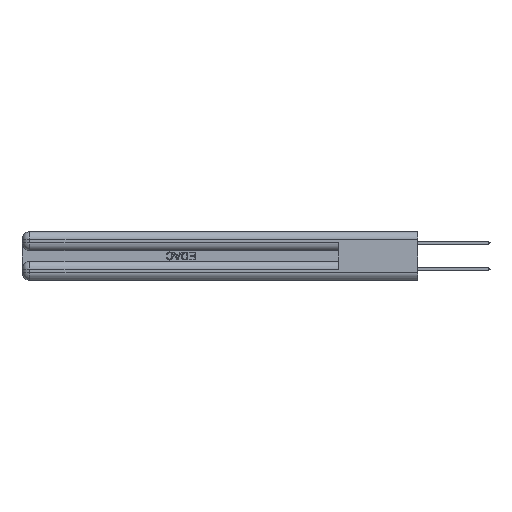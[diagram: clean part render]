
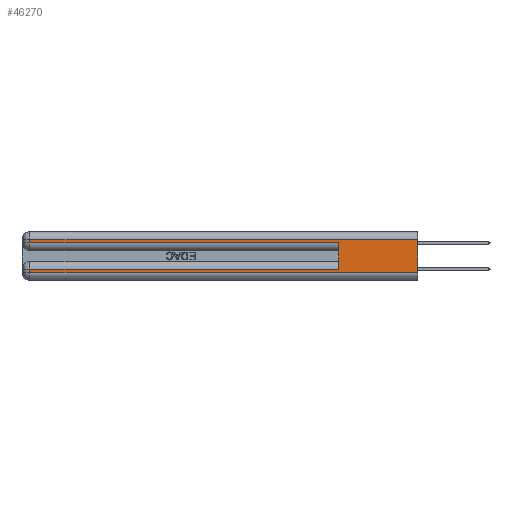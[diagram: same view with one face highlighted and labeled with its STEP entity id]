
A CAD part, left-side view. The second image highlights one B-rep face of the part: STEP entity #46270.
In plain terms, the highlighted planar face has unit normal (-1, 0, 0).
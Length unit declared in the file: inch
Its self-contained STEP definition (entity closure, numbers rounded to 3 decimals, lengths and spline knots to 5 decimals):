
#1334 = CARTESIAN_POINT ( 'NONE',  ( 0., 2.94, 0.085 ) ) ;
#1571 = DIRECTION ( 'NONE',  ( 1., 0., 0. ) ) ;
#2046 = VECTOR ( 'NONE', #31151, 39.37008 ) ;
#2434 = AXIS2_PLACEMENT_3D ( 'NONE', #24019, #1571, #27946 ) ;
#3296 = LINE ( 'NONE', #25047, #31011 ) ;
#3628 = EDGE_LOOP ( 'NONE', ( #4961, #23378, #37711, #9374, #30080, #7433, #8274, #8623 ) ) ;
#3970 = DIRECTION ( 'NONE',  ( 0., 0., -1. ) ) ;
#4219 = EDGE_CURVE ( 'NONE', #15027, #23163, #40047, .T. ) ;
#4768 = CARTESIAN_POINT ( 'NONE',  ( 0., 0., 0.285 ) ) ;
#4961 = ORIENTED_EDGE ( 'NONE', *, *, #28759, .F. ) ;
#6070 = DIRECTION ( 'NONE',  ( 0., 1., 0. ) ) ;
#7433 = ORIENTED_EDGE ( 'NONE', *, *, #25814, .T. ) ;
#7521 = CARTESIAN_POINT ( 'NONE',  ( 0., 0.6, 0.085 ) ) ;
#8274 = ORIENTED_EDGE ( 'NONE', *, *, #43996, .T. ) ;
#8623 = ORIENTED_EDGE ( 'NONE', *, *, #4219, .T. ) ;
#9374 = ORIENTED_EDGE ( 'NONE', *, *, #42820, .T. ) ;
#12802 = CARTESIAN_POINT ( 'NONE',  ( 0., 0., 0.31 ) ) ;
#14272 = LINE ( 'NONE', #15020, #41834 ) ;
#15020 = CARTESIAN_POINT ( 'NONE',  ( 0., 0., 0.37 ) ) ;
#15027 = VERTEX_POINT ( 'NONE', #15856 ) ;
#15388 = CARTESIAN_POINT ( 'NONE',  ( 0., 0., 0.06 ) ) ;
#15402 = DIRECTION ( 'NONE',  ( 0., 0., -1. ) ) ;
#15676 = LINE ( 'NONE', #45189, #44361 ) ;
#15723 = LINE ( 'NONE', #34809, #43228 ) ;
#15856 = CARTESIAN_POINT ( 'NONE',  ( 0., 2.94, 0.06 ) ) ;
#16581 = VERTEX_POINT ( 'NONE', #17724 ) ;
#16589 = DIRECTION ( 'NONE',  ( 0., 1., 0. ) ) ;
#17169 = VECTOR ( 'NONE', #43447, 39.37008 ) ;
#17310 = CARTESIAN_POINT ( 'NONE',  ( 0., 2.94, 0.37 ) ) ;
#17724 = CARTESIAN_POINT ( 'NONE',  ( 0., 0., 0.31 ) ) ;
#20739 = EDGE_CURVE ( 'NONE', #16581, #26210, #39773, .T. ) ;
#21359 = VERTEX_POINT ( 'NONE', #27719 ) ;
#23163 = VERTEX_POINT ( 'NONE', #15388 ) ;
#23378 = ORIENTED_EDGE ( 'NONE', *, *, #20739, .T. ) ;
#23941 = EDGE_CURVE ( 'NONE', #26210, #21359, #26007, .T. ) ;
#24019 = CARTESIAN_POINT ( 'NONE',  ( 0., 0., 0.37 ) ) ;
#24650 = CARTESIAN_POINT ( 'NONE',  ( 0., 0., 0.06 ) ) ;
#25047 = CARTESIAN_POINT ( 'NONE',  ( 0., 0., 0.085 ) ) ;
#25814 = EDGE_CURVE ( 'NONE', #48408, #33801, #3296, .T. ) ;
#26007 = LINE ( 'NONE', #17310, #17169 ) ;
#26210 = VERTEX_POINT ( 'NONE', #27298 ) ;
#27298 = CARTESIAN_POINT ( 'NONE',  ( 0., 2.94, 0.31 ) ) ;
#27719 = CARTESIAN_POINT ( 'NONE',  ( 0., 2.94, 0.285 ) ) ;
#27946 = DIRECTION ( 'NONE',  ( 0., 0., -1. ) ) ;
#28481 = FACE_OUTER_BOUND ( 'NONE', #3628, .T. ) ;
#28759 = EDGE_CURVE ( 'NONE', #16581, #23163, #14272, .T. ) ;
#29765 = LINE ( 'NONE', #4768, #2046 ) ;
#30080 = ORIENTED_EDGE ( 'NONE', *, *, #43512, .F. ) ;
#30147 = VECTOR ( 'NONE', #43397, 39.37008 ) ;
#31011 = VECTOR ( 'NONE', #6070, 39.37008 ) ;
#31151 = DIRECTION ( 'NONE',  ( 0., -1., 0. ) ) ;
#33801 = VERTEX_POINT ( 'NONE', #1334 ) ;
#34809 = CARTESIAN_POINT ( 'NONE',  ( 0., 0.6, 0.145 ) ) ;
#37660 = CARTESIAN_POINT ( 'NONE',  ( 0., 0.6, 0.285 ) ) ;
#37711 = ORIENTED_EDGE ( 'NONE', *, *, #23941, .T. ) ;
#39773 = LINE ( 'NONE', #12802, #48494 ) ;
#40047 = LINE ( 'NONE', #24650, #30147 ) ;
#41834 = VECTOR ( 'NONE', #3970, 39.37008 ) ;
#42820 = EDGE_CURVE ( 'NONE', #21359, #45348, #29765, .T. ) ;
#43228 = VECTOR ( 'NONE', #46039, 39.37008 ) ;
#43397 = DIRECTION ( 'NONE',  ( 0., -1., 0. ) ) ;
#43447 = DIRECTION ( 'NONE',  ( 0., 0., -1. ) ) ;
#43512 = EDGE_CURVE ( 'NONE', #48408, #45348, #15723, .T. ) ;
#43996 = EDGE_CURVE ( 'NONE', #33801, #15027, #15676, .T. ) ;
#44361 = VECTOR ( 'NONE', #15402, 39.37008 ) ;
#45189 = CARTESIAN_POINT ( 'NONE',  ( 0., 2.94, 0.37 ) ) ;
#45348 = VERTEX_POINT ( 'NONE', #37660 ) ;
#46039 = DIRECTION ( 'NONE',  ( 0., 0., 1. ) ) ;
#46270 = ADVANCED_FACE ( 'NONE', ( #28481 ), #46521, .F. ) ;
#46521 = PLANE ( 'NONE',  #2434 ) ;
#48408 = VERTEX_POINT ( 'NONE', #7521 ) ;
#48494 = VECTOR ( 'NONE', #16589, 39.37008 ) ;
